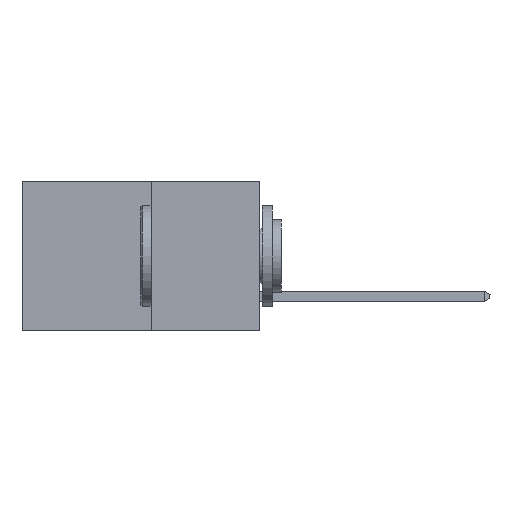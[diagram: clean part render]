
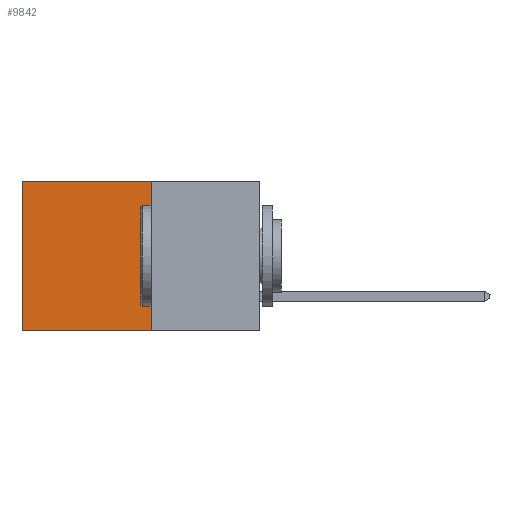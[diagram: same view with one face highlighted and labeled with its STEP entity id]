
A CAD part, left-side view. The second image highlights one B-rep face of the part: STEP entity #9842.
In plain terms, the highlighted planar face has unit normal (-1, 0, 0).
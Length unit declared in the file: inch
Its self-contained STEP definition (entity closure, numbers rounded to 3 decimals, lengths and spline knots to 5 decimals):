
#181 = CARTESIAN_POINT ( 'NONE',  ( 0.277, 0.27, -0.37 ) ) ;
#325 = DIRECTION ( 'NONE',  ( 0., 0., -1. ) ) ;
#337 = LINE ( 'NONE', #5885, #8446 ) ;
#418 = FACE_OUTER_BOUND ( 'NONE', #8833, .T. ) ;
#686 = EDGE_CURVE ( 'NONE', #2175, #4804, #3191, .T. ) ;
#989 = VECTOR ( 'NONE', #4653, 39.37008 ) ;
#1000 = DIRECTION ( 'NONE',  ( 0., 0., -1. ) ) ;
#1251 = CARTESIAN_POINT ( 'NONE',  ( 0.277, 0.27, -0.37 ) ) ;
#1530 = EDGE_CURVE ( 'NONE', #4804, #6566, #7974, .T. ) ;
#1656 = CARTESIAN_POINT ( 'NONE',  ( 0.277, 0.59, 0. ) ) ;
#2105 = ORIENTED_EDGE ( 'NONE', *, *, #8018, .T. ) ;
#2175 = VERTEX_POINT ( 'NONE', #8595 ) ;
#3191 = LINE ( 'NONE', #1251, #989 ) ;
#3447 = PLANE ( 'NONE',  #3955 ) ;
#3630 = CARTESIAN_POINT ( 'NONE',  ( 0.277, 0.27, 0. ) ) ;
#3829 = VERTEX_POINT ( 'NONE', #1656 ) ;
#3955 = AXIS2_PLACEMENT_3D ( 'NONE', #181, #5743, #1000 ) ;
#4109 = EDGE_CURVE ( 'NONE', #2175, #3829, #9004, .T. ) ;
#4653 = DIRECTION ( 'NONE',  ( 0., 0., -1. ) ) ;
#4769 = DIRECTION ( 'NONE',  ( 0., 1., 0. ) ) ;
#4804 = VERTEX_POINT ( 'NONE', #9503 ) ;
#5190 = VECTOR ( 'NONE', #4769, 39.37008 ) ;
#5372 = CARTESIAN_POINT ( 'NONE',  ( 0.277, 0.59, -0.37 ) ) ;
#5743 = DIRECTION ( 'NONE',  ( 1., 0., 0. ) ) ;
#5885 = CARTESIAN_POINT ( 'NONE',  ( 0.277, 0.59, -0.37 ) ) ;
#5927 = VECTOR ( 'NONE', #9657, 39.37008 ) ;
#6394 = ORIENTED_EDGE ( 'NONE', *, *, #4109, .T. ) ;
#6566 = VERTEX_POINT ( 'NONE', #5372 ) ;
#6982 = ORIENTED_EDGE ( 'NONE', *, *, #1530, .F. ) ;
#7121 = CARTESIAN_POINT ( 'NONE',  ( 0.277, 0.27, -0.37 ) ) ;
#7974 = LINE ( 'NONE', #7121, #5927 ) ;
#8018 = EDGE_CURVE ( 'NONE', #3829, #6566, #337, .T. ) ;
#8446 = VECTOR ( 'NONE', #325, 39.37008 ) ;
#8595 = CARTESIAN_POINT ( 'NONE',  ( 0.277, 0.27, 0. ) ) ;
#8833 = EDGE_LOOP ( 'NONE', ( #2105, #6982, #9732, #6394 ) ) ;
#9004 = LINE ( 'NONE', #3630, #5190 ) ;
#9503 = CARTESIAN_POINT ( 'NONE',  ( 0.277, 0.27, -0.37 ) ) ;
#9657 = DIRECTION ( 'NONE',  ( 0., 1., 0. ) ) ;
#9732 = ORIENTED_EDGE ( 'NONE', *, *, #686, .F. ) ;
#9842 = ADVANCED_FACE ( 'NONE', ( #418 ), #3447, .F. ) ;
